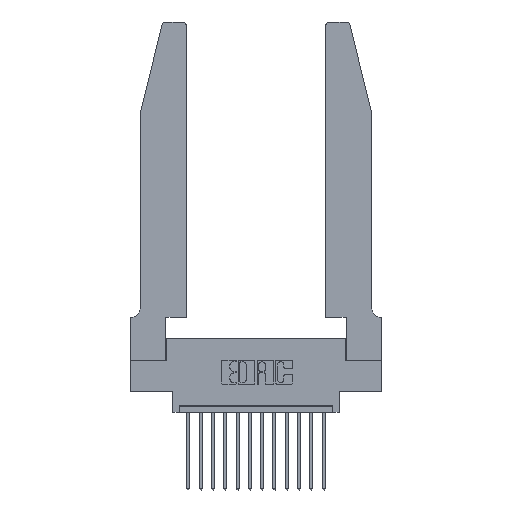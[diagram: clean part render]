
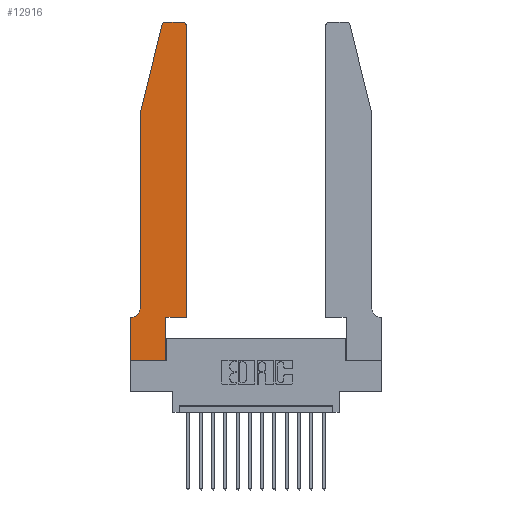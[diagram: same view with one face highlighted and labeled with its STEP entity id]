
A CAD part, top view. The second image highlights one B-rep face of the part: STEP entity #12916.
In plain terms, the highlighted planar face has unit normal (0, 0, 1).
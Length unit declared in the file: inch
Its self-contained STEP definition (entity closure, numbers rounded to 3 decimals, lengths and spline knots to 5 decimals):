
#638 = DIRECTION ( 'NONE',  ( 1., 0., 0. ) ) ;
#726 = VERTEX_POINT ( 'NONE', #2871 ) ;
#1008 = VERTEX_POINT ( 'NONE', #2230 ) ;
#1138 = CARTESIAN_POINT ( 'NONE',  ( 0.0055, 0.42, 0.37 ) ) ;
#1523 = LINE ( 'NONE', #11471, #17357 ) ;
#1535 = DIRECTION ( 'NONE',  ( 1., 0., 0. ) ) ;
#1656 = CARTESIAN_POINT ( 'NONE',  ( 0., 0., 0.37 ) ) ;
#1694 = CARTESIAN_POINT ( 'NONE',  ( 0.4505, 0.35, 0.37 ) ) ;
#1703 = DIRECTION ( 'NONE',  ( 0., 0., 1. ) ) ;
#1769 = DIRECTION ( 'NONE',  ( 1., 0., 0. ) ) ;
#2113 = CARTESIAN_POINT ( 'NONE',  ( 0.2865, 0., 0.37 ) ) ;
#2230 = CARTESIAN_POINT ( 'NONE',  ( 0.4505, 0.35, 0.37 ) ) ;
#2291 = DIRECTION ( 'NONE',  ( 0., 1., 0. ) ) ;
#2425 = VERTEX_POINT ( 'NONE', #13044 ) ;
#2466 = EDGE_CURVE ( 'NONE', #11334, #13608, #2647, .T. ) ;
#2468 = DIRECTION ( 'NONE',  ( -1., 0., 0. ) ) ;
#2647 = CIRCLE ( 'NONE', #4389, 0.07 ) ;
#2871 = CARTESIAN_POINT ( 'NONE',  ( 0., 0.35, 0.37 ) ) ;
#3123 = ORIENTED_EDGE ( 'NONE', *, *, #13095, .T. ) ;
#3156 = PLANE ( 'NONE',  #8802 ) ;
#3262 = EDGE_CURVE ( 'NONE', #15152, #4610, #4781, .T. ) ;
#3354 = EDGE_CURVE ( 'NONE', #17856, #14232, #6926, .T. ) ;
#3576 = DIRECTION ( 'NONE',  ( 1., 0., 0. ) ) ;
#3606 = CARTESIAN_POINT ( 'NONE',  ( 0.0755, 0.42, 0.37 ) ) ;
#4168 = CARTESIAN_POINT ( 'NONE',  ( 0.0755, 2., 0.37 ) ) ;
#4389 = AXIS2_PLACEMENT_3D ( 'NONE', #1138, #15052, #2468 ) ;
#4610 = VERTEX_POINT ( 'NONE', #11877 ) ;
#4743 = DIRECTION ( 'NONE',  ( 0., 0., 1. ) ) ;
#4781 = LINE ( 'NONE', #5915, #15394 ) ;
#5412 = EDGE_CURVE ( 'NONE', #13519, #12562, #5894, .T. ) ;
#5688 = DIRECTION ( 'NONE',  ( 0., 0., 1. ) ) ;
#5694 = ORIENTED_EDGE ( 'NONE', *, *, #2466, .T. ) ;
#5720 = ORIENTED_EDGE ( 'NONE', *, *, #3354, .T. ) ;
#5754 = CARTESIAN_POINT ( 'NONE',  ( 0.4505, 2.72, 0.37 ) ) ;
#5894 = LINE ( 'NONE', #1656, #14116 ) ;
#5915 = CARTESIAN_POINT ( 'NONE',  ( 0.0755, 2., 0.37 ) ) ;
#6018 = ORIENTED_EDGE ( 'NONE', *, *, #12797, .T. ) ;
#6178 = EDGE_CURVE ( 'NONE', #1008, #17856, #11501, .T. ) ;
#6440 = ORIENTED_EDGE ( 'NONE', *, *, #7698, .T. ) ;
#6656 = FACE_OUTER_BOUND ( 'NONE', #7566, .T. ) ;
#6751 = DIRECTION ( 'NONE',  ( -0.239, -0.971, 0. ) ) ;
#6926 = CIRCLE ( 'NONE', #7884, 0.03 ) ;
#7104 = DIRECTION ( 'NONE',  ( 0., -1., 0. ) ) ;
#7278 = ORIENTED_EDGE ( 'NONE', *, *, #8151, .T. ) ;
#7566 = EDGE_LOOP ( 'NONE', ( #3123, #11482, #7921, #6018, #5694, #7278, #14344, #12908, #13897, #6440, #10089, #5720 ) ) ;
#7585 = VERTEX_POINT ( 'NONE', #14531 ) ;
#7698 = EDGE_CURVE ( 'NONE', #7585, #1008, #17809, .T. ) ;
#7884 = AXIS2_PLACEMENT_3D ( 'NONE', #9908, #1703, #17054 ) ;
#7921 = ORIENTED_EDGE ( 'NONE', *, *, #3262, .T. ) ;
#8037 = LINE ( 'NONE', #8993, #8477 ) ;
#8145 = CARTESIAN_POINT ( 'NONE',  ( 0.25487, 2.72718, 0.37 ) ) ;
#8151 = EDGE_CURVE ( 'NONE', #13608, #726, #1523, .T. ) ;
#8362 = CARTESIAN_POINT ( 'NONE',  ( 0., 0., 0.37 ) ) ;
#8438 = CIRCLE ( 'NONE', #11044, 0.03 ) ;
#8477 = VECTOR ( 'NONE', #2291, 39.37008 ) ;
#8514 = CARTESIAN_POINT ( 'NONE',  ( 0., 0.35, 0.37 ) ) ;
#8551 = DIRECTION ( 'NONE',  ( -1., 0., 0. ) ) ;
#8592 = VECTOR ( 'NONE', #17962, 39.37008 ) ;
#8802 = AXIS2_PLACEMENT_3D ( 'NONE', #8514, #5688, #1535 ) ;
#8887 = CARTESIAN_POINT ( 'NONE',  ( 0.2605, 2.75, 0.37 ) ) ;
#8993 = CARTESIAN_POINT ( 'NONE',  ( 0.2865, 0.35, 0.37 ) ) ;
#9056 = CARTESIAN_POINT ( 'NONE',  ( 0.0055, 0.35, 0.37 ) ) ;
#9074 = CARTESIAN_POINT ( 'NONE',  ( 0.4505, 0.35, 0.37 ) ) ;
#9908 = CARTESIAN_POINT ( 'NONE',  ( 0.4205, 2.72, 0.37 ) ) ;
#10089 = ORIENTED_EDGE ( 'NONE', *, *, #6178, .T. ) ;
#10198 = VECTOR ( 'NONE', #7104, 39.37008 ) ;
#10374 = LINE ( 'NONE', #8887, #15129 ) ;
#10839 = LINE ( 'NONE', #13828, #10198 ) ;
#11044 = AXIS2_PLACEMENT_3D ( 'NONE', #17270, #4743, #638 ) ;
#11334 = VERTEX_POINT ( 'NONE', #3606 ) ;
#11471 = CARTESIAN_POINT ( 'NONE',  ( 0.0755, 0.35, 0.37 ) ) ;
#11482 = ORIENTED_EDGE ( 'NONE', *, *, #17539, .T. ) ;
#11501 = LINE ( 'NONE', #1694, #14795 ) ;
#11568 = DIRECTION ( 'NONE',  ( -1., 0., 0. ) ) ;
#11683 = EDGE_CURVE ( 'NONE', #726, #13519, #10839, .T. ) ;
#11877 = CARTESIAN_POINT ( 'NONE',  ( 0.0755, 2., 0.37 ) ) ;
#12562 = VERTEX_POINT ( 'NONE', #2113 ) ;
#12797 = EDGE_CURVE ( 'NONE', #4610, #11334, #14925, .T. ) ;
#12908 = ORIENTED_EDGE ( 'NONE', *, *, #5412, .T. ) ;
#12916 = ADVANCED_FACE ( 'NONE', ( #6656 ), #3156, .T. ) ;
#13044 = CARTESIAN_POINT ( 'NONE',  ( 0.284, 2.75, 0.37 ) ) ;
#13095 = EDGE_CURVE ( 'NONE', #14232, #2425, #10374, .T. ) ;
#13519 = VERTEX_POINT ( 'NONE', #8362 ) ;
#13608 = VERTEX_POINT ( 'NONE', #9056 ) ;
#13828 = CARTESIAN_POINT ( 'NONE',  ( 0., 0., 0.37 ) ) ;
#13897 = ORIENTED_EDGE ( 'NONE', *, *, #16210, .T. ) ;
#14116 = VECTOR ( 'NONE', #1769, 39.37008 ) ;
#14232 = VERTEX_POINT ( 'NONE', #17285 ) ;
#14344 = ORIENTED_EDGE ( 'NONE', *, *, #11683, .T. ) ;
#14531 = CARTESIAN_POINT ( 'NONE',  ( 0.2865, 0.35, 0.37 ) ) ;
#14795 = VECTOR ( 'NONE', #15309, 39.37008 ) ;
#14925 = LINE ( 'NONE', #4168, #8592 ) ;
#15052 = DIRECTION ( 'NONE',  ( 0., 0., -1. ) ) ;
#15129 = VECTOR ( 'NONE', #11568, 39.37008 ) ;
#15152 = VERTEX_POINT ( 'NONE', #8145 ) ;
#15309 = DIRECTION ( 'NONE',  ( 0., 1., 0. ) ) ;
#15394 = VECTOR ( 'NONE', #6751, 39.37008 ) ;
#16210 = EDGE_CURVE ( 'NONE', #12562, #7585, #8037, .T. ) ;
#17054 = DIRECTION ( 'NONE',  ( 1., 0., 0. ) ) ;
#17270 = CARTESIAN_POINT ( 'NONE',  ( 0.284, 2.72, 0.37 ) ) ;
#17285 = CARTESIAN_POINT ( 'NONE',  ( 0.4205, 2.75, 0.37 ) ) ;
#17357 = VECTOR ( 'NONE', #8551, 39.37008 ) ;
#17539 = EDGE_CURVE ( 'NONE', #2425, #15152, #8438, .T. ) ;
#17576 = VECTOR ( 'NONE', #3576, 39.37008 ) ;
#17809 = LINE ( 'NONE', #9074, #17576 ) ;
#17856 = VERTEX_POINT ( 'NONE', #5754 ) ;
#17962 = DIRECTION ( 'NONE',  ( 0., -1., 0. ) ) ;
